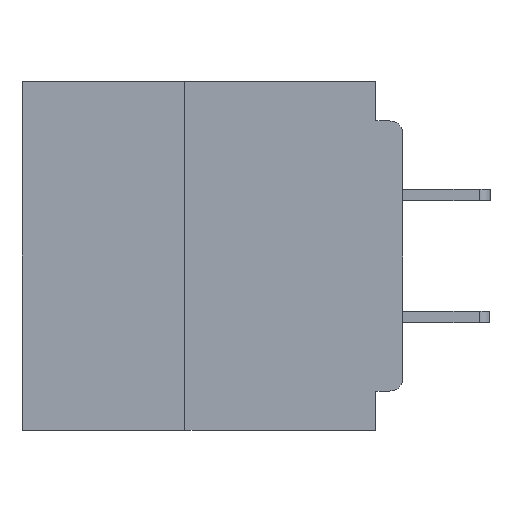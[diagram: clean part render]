
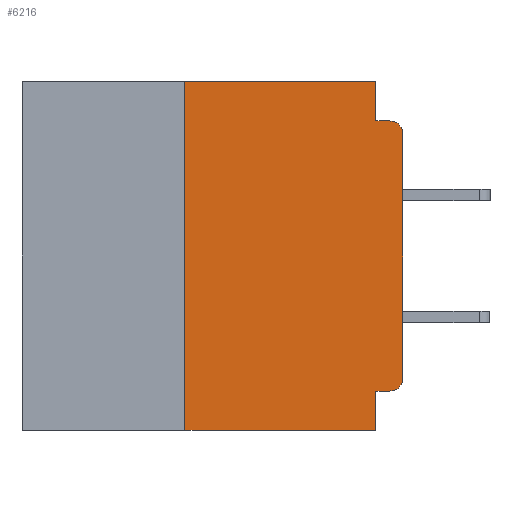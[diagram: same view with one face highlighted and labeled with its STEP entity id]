
A CAD part, left-side view. The second image highlights one B-rep face of the part: STEP entity #6216.
In plain terms, the highlighted planar face has unit normal (-1, 0, 0).
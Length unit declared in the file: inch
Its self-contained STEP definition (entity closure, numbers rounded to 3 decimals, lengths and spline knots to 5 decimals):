
#322 = CIRCLE ( 'NONE', #15099, 0.015 ) ;
#399 = AXIS2_PLACEMENT_3D ( 'NONE', #15762, #45547, #20048 ) ;
#1448 = CARTESIAN_POINT ( 'NONE',  ( 0., 0., 0. ) ) ;
#2299 = CARTESIAN_POINT ( 'NONE',  ( 0., 0.031, -0.045 ) ) ;
#2989 = VECTOR ( 'NONE', #13659, 39.37008 ) ;
#5118 = EDGE_CURVE ( 'NONE', #43419, #8177, #53880, .T. ) ;
#5590 = DIRECTION ( 'NONE',  ( 0., 0., -1. ) ) ;
#5779 = CARTESIAN_POINT ( 'NONE',  ( 0., 0.031, -0.4 ) ) ;
#6216 = ADVANCED_FACE ( 'NONE', ( #45046 ), #42577, .F. ) ;
#6466 = EDGE_CURVE ( 'NONE', #22725, #21703, #20391, .T. ) ;
#7192 = ORIENTED_EDGE ( 'NONE', *, *, #34305, .F. ) ;
#7554 = EDGE_CURVE ( 'NONE', #42427, #41370, #33583, .T. ) ;
#8177 = VERTEX_POINT ( 'NONE', #29614 ) ;
#8419 = LINE ( 'NONE', #23737, #41048 ) ;
#8611 = EDGE_CURVE ( 'NONE', #21703, #41370, #46195, .T. ) ;
#9057 = VECTOR ( 'NONE', #47422, 39.37008 ) ;
#9478 = EDGE_CURVE ( 'NONE', #30272, #49975, #24758, .T. ) ;
#10750 = DIRECTION ( 'NONE',  ( 0., -1., 0. ) ) ;
#12522 = CARTESIAN_POINT ( 'NONE',  ( 0., 0.015, -0.045 ) ) ;
#12744 = CARTESIAN_POINT ( 'NONE',  ( 0., 0., -0.355 ) ) ;
#13432 = ORIENTED_EDGE ( 'NONE', *, *, #8611, .T. ) ;
#13659 = DIRECTION ( 'NONE',  ( 0., 0., -1. ) ) ;
#14369 = LINE ( 'NONE', #43447, #2989 ) ;
#15099 = AXIS2_PLACEMENT_3D ( 'NONE', #16267, #46045, #20555 ) ;
#15762 = CARTESIAN_POINT ( 'NONE',  ( 0., 0.015, -0.06 ) ) ;
#16267 = CARTESIAN_POINT ( 'NONE',  ( 0., 0.015, -0.34 ) ) ;
#17442 = ORIENTED_EDGE ( 'NONE', *, *, #5118, .T. ) ;
#20048 = DIRECTION ( 'NONE',  ( 0., 0., -1. ) ) ;
#20391 = LINE ( 'NONE', #1448, #9057 ) ;
#20555 = DIRECTION ( 'NONE',  ( 0., 0., -1. ) ) ;
#20590 = ORIENTED_EDGE ( 'NONE', *, *, #7554, .F. ) ;
#21703 = VERTEX_POINT ( 'NONE', #45618 ) ;
#22725 = VERTEX_POINT ( 'NONE', #31547 ) ;
#23323 = EDGE_CURVE ( 'NONE', #29635, #8177, #54892, .T. ) ;
#23636 = VECTOR ( 'NONE', #5590, 39.37008 ) ;
#23737 = CARTESIAN_POINT ( 'NONE',  ( 0., 0.25, -0.4 ) ) ;
#24453 = ORIENTED_EDGE ( 'NONE', *, *, #9478, .F. ) ;
#24605 = CARTESIAN_POINT ( 'NONE',  ( 0., 0., -0.045 ) ) ;
#24758 = LINE ( 'NONE', #31992, #46078 ) ;
#24864 = CARTESIAN_POINT ( 'NONE',  ( 0., 0.031, 0. ) ) ;
#25583 = DIRECTION ( 'NONE',  ( 0., 0., -1. ) ) ;
#26083 = CARTESIAN_POINT ( 'NONE',  ( 0., 0.031, -0.355 ) ) ;
#26883 = CARTESIAN_POINT ( 'NONE',  ( 0., 0.015, -0.355 ) ) ;
#27045 = EDGE_LOOP ( 'NONE', ( #38676, #13432, #20590, #35249, #24453, #41897, #17442, #46775, #7192, #33745 ) ) ;
#28926 = DIRECTION ( 'NONE',  ( 0., -1., 0. ) ) ;
#29614 = CARTESIAN_POINT ( 'NONE',  ( 0., 0.031, -0.4 ) ) ;
#29635 = VERTEX_POINT ( 'NONE', #26083 ) ;
#29966 = VECTOR ( 'NONE', #46939, 39.37008 ) ;
#30272 = VERTEX_POINT ( 'NONE', #45405 ) ;
#31547 = CARTESIAN_POINT ( 'NONE',  ( 0., 0., -0.34 ) ) ;
#31992 = CARTESIAN_POINT ( 'NONE',  ( 0., 0.437, 0. ) ) ;
#33583 = LINE ( 'NONE', #24605, #44877 ) ;
#33745 = ORIENTED_EDGE ( 'NONE', *, *, #41065, .T. ) ;
#34305 = EDGE_CURVE ( 'NONE', #38928, #29635, #42855, .T. ) ;
#35249 = ORIENTED_EDGE ( 'NONE', *, *, #53619, .F. ) ;
#38327 = DIRECTION ( 'NONE',  ( 0., 1., 0. ) ) ;
#38676 = ORIENTED_EDGE ( 'NONE', *, *, #6466, .T. ) ;
#38928 = VERTEX_POINT ( 'NONE', #26883 ) ;
#41048 = VECTOR ( 'NONE', #44966, 39.37008 ) ;
#41065 = EDGE_CURVE ( 'NONE', #38928, #22725, #322, .T. ) ;
#41370 = VERTEX_POINT ( 'NONE', #12522 ) ;
#41526 = VECTOR ( 'NONE', #38327, 39.37008 ) ;
#41897 = ORIENTED_EDGE ( 'NONE', *, *, #45099, .F. ) ;
#42427 = VERTEX_POINT ( 'NONE', #2299 ) ;
#42577 = PLANE ( 'NONE',  #50026 ) ;
#42855 = LINE ( 'NONE', #12744, #41526 ) ;
#43419 = VERTEX_POINT ( 'NONE', #52519 ) ;
#43447 = CARTESIAN_POINT ( 'NONE',  ( 0., 0.031, 0. ) ) ;
#44877 = VECTOR ( 'NONE', #28926, 39.37008 ) ;
#44966 = DIRECTION ( 'NONE',  ( 0., 0., 1. ) ) ;
#45046 = FACE_OUTER_BOUND ( 'NONE', #27045, .T. ) ;
#45099 = EDGE_CURVE ( 'NONE', #43419, #30272, #8419, .T. ) ;
#45405 = CARTESIAN_POINT ( 'NONE',  ( 0., 0.25, 0. ) ) ;
#45547 = DIRECTION ( 'NONE',  ( -1., 0., 0. ) ) ;
#45618 = CARTESIAN_POINT ( 'NONE',  ( 0., 0., -0.06 ) ) ;
#46045 = DIRECTION ( 'NONE',  ( -1., 0., 0. ) ) ;
#46078 = VECTOR ( 'NONE', #10750, 39.37008 ) ;
#46195 = CIRCLE ( 'NONE', #399, 0.015 ) ;
#46775 = ORIENTED_EDGE ( 'NONE', *, *, #23323, .F. ) ;
#46939 = DIRECTION ( 'NONE',  ( 0., -1., 0. ) ) ;
#47422 = DIRECTION ( 'NONE',  ( 0., 0., 1. ) ) ;
#49975 = VERTEX_POINT ( 'NONE', #24864 ) ;
#50026 = AXIS2_PLACEMENT_3D ( 'NONE', #55139, #51094, #25583 ) ;
#51094 = DIRECTION ( 'NONE',  ( 1., 0., 0. ) ) ;
#51389 = CARTESIAN_POINT ( 'NONE',  ( 0., 0.437, -0.4 ) ) ;
#52519 = CARTESIAN_POINT ( 'NONE',  ( 0., 0.25, -0.4 ) ) ;
#53619 = EDGE_CURVE ( 'NONE', #49975, #42427, #14369, .T. ) ;
#53880 = LINE ( 'NONE', #51389, #29966 ) ;
#54892 = LINE ( 'NONE', #5779, #23636 ) ;
#55139 = CARTESIAN_POINT ( 'NONE',  ( 0., 0.437, 0. ) ) ;
